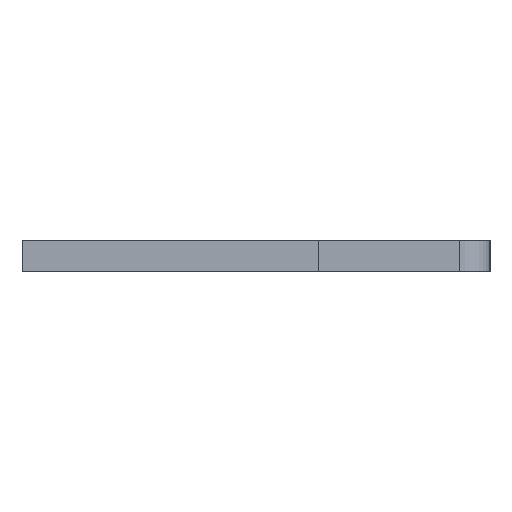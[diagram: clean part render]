
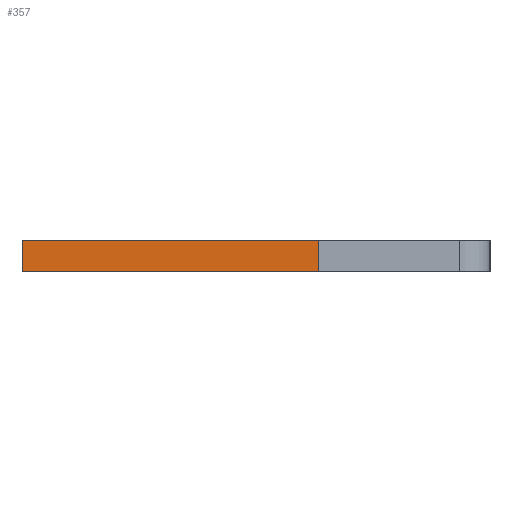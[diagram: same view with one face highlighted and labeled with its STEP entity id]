
A CAD part, left-side view. The second image highlights one B-rep face of the part: STEP entity #357.
In plain terms, the highlighted face is planar.
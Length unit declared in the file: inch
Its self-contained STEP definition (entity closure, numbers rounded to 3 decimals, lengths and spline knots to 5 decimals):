
#14 = DIRECTION ( 'NONE',  ( 0., 1., 0. ) ) ;
#59 = VECTOR ( 'NONE', #919, 39.37008 ) ;
#154 = DIRECTION ( 'NONE',  ( 0., 0., 1. ) ) ;
#160 = VECTOR ( 'NONE', #1309, 39.37008 ) ;
#162 = EDGE_CURVE ( 'NONE', #442, #380, #188, .T. ) ;
#186 = LINE ( 'NONE', #451, #160 ) ;
#188 = LINE ( 'NONE', #1118, #418 ) ;
#202 = DIRECTION ( 'NONE',  ( 0., 1., 0. ) ) ;
#221 = LINE ( 'NONE', #1037, #59 ) ;
#293 = CARTESIAN_POINT ( 'NONE',  ( -0.01, -0.04, -0.04 ) ) ;
#305 = CARTESIAN_POINT ( 'NONE',  ( -0.01, 0.15, -0.04 ) ) ;
#337 = ORIENTED_EDGE ( 'NONE', *, *, #1123, .T. ) ;
#357 = ADVANCED_FACE ( 'NONE', ( #1577 ), #1545, .F. ) ;
#380 = VERTEX_POINT ( 'NONE', #305 ) ;
#418 = VECTOR ( 'NONE', #14, 39.37008 ) ;
#429 = CARTESIAN_POINT ( 'NONE',  ( 0.01, 0.15, -0.04 ) ) ;
#442 = VERTEX_POINT ( 'NONE', #293 ) ;
#445 = ORIENTED_EDGE ( 'NONE', *, *, #825, .F. ) ;
#451 = CARTESIAN_POINT ( 'NONE',  ( 0.01, 0.15, -0.04 ) ) ;
#459 = EDGE_LOOP ( 'NONE', ( #941, #445, #1364, #337 ) ) ;
#731 = AXIS2_PLACEMENT_3D ( 'NONE', #429, #154, #1672 ) ;
#825 = EDGE_CURVE ( 'NONE', #1276, #380, #186, .T. ) ;
#919 = DIRECTION ( 'NONE',  ( -1., 0., 0. ) ) ;
#941 = ORIENTED_EDGE ( 'NONE', *, *, #162, .T. ) ;
#1037 = CARTESIAN_POINT ( 'NONE',  ( 0.01, -0.04, -0.04 ) ) ;
#1118 = CARTESIAN_POINT ( 'NONE',  ( -0.01, 0.15, -0.04 ) ) ;
#1123 = EDGE_CURVE ( 'NONE', #1392, #442, #221, .T. ) ;
#1176 = CARTESIAN_POINT ( 'NONE',  ( 0.01, 0.15, -0.04 ) ) ;
#1193 = VECTOR ( 'NONE', #202, 39.37008 ) ;
#1198 = CARTESIAN_POINT ( 'NONE',  ( 0.01, -0.04, -0.04 ) ) ;
#1204 = CARTESIAN_POINT ( 'NONE',  ( 0.01, 0.15, -0.04 ) ) ;
#1266 = EDGE_CURVE ( 'NONE', #1392, #1276, #1304, .T. ) ;
#1276 = VERTEX_POINT ( 'NONE', #1176 ) ;
#1304 = LINE ( 'NONE', #1204, #1193 ) ;
#1309 = DIRECTION ( 'NONE',  ( -1., 0., 0. ) ) ;
#1364 = ORIENTED_EDGE ( 'NONE', *, *, #1266, .F. ) ;
#1392 = VERTEX_POINT ( 'NONE', #1198 ) ;
#1545 = PLANE ( 'NONE',  #731 ) ;
#1577 = FACE_OUTER_BOUND ( 'NONE', #459, .T. ) ;
#1672 = DIRECTION ( 'NONE',  ( 1., 0., 0. ) ) ;
